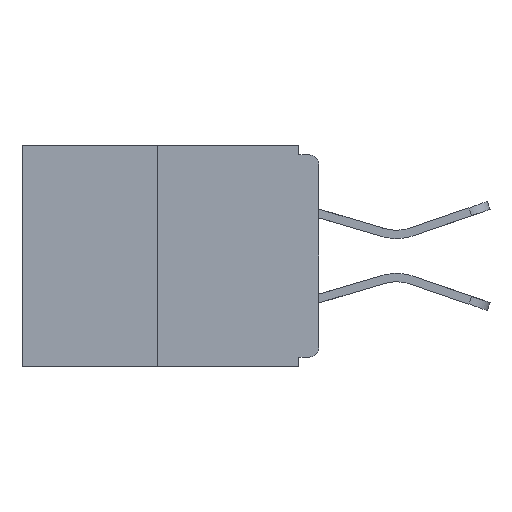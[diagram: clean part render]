
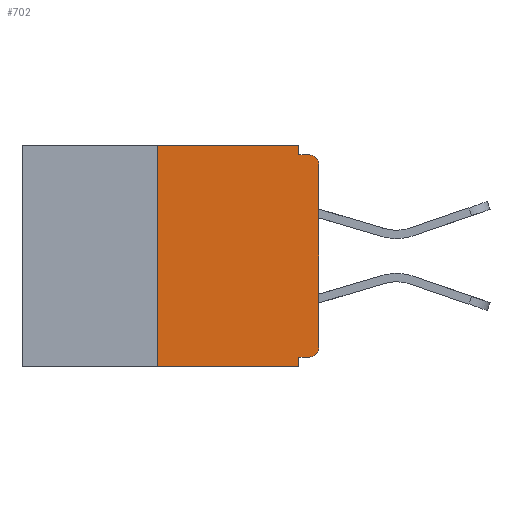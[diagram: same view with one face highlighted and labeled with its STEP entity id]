
A CAD part, left-side view. The second image highlights one B-rep face of the part: STEP entity #702.
In plain terms, the highlighted planar face has unit normal (-1, 0, 0).
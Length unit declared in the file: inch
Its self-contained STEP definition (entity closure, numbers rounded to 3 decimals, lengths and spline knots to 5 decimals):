
#124 = ORIENTED_EDGE ( 'NONE', *, *, #10964, .F. ) ;
#320 = VERTEX_POINT ( 'NONE', #9749 ) ;
#351 = PLANE ( 'NONE',  #2901 ) ;
#610 = ORIENTED_EDGE ( 'NONE', *, *, #4471, .F. ) ;
#689 = CARTESIAN_POINT ( 'NONE',  ( 0., 0., 0. ) ) ;
#702 = ADVANCED_FACE ( 'NONE', ( #7585 ), #351, .F. ) ;
#805 = VERTEX_POINT ( 'NONE', #10018 ) ;
#1058 = CARTESIAN_POINT ( 'NONE',  ( 0., 0.015, -0.313 ) ) ;
#1541 = VECTOR ( 'NONE', #9274, 39.37008 ) ;
#1599 = LINE ( 'NONE', #11029, #1541 ) ;
#1915 = LINE ( 'NONE', #8311, #6901 ) ;
#1949 = DIRECTION ( 'NONE',  ( 0., -1., 0. ) ) ;
#2059 = VERTEX_POINT ( 'NONE', #11018 ) ;
#2078 = EDGE_CURVE ( 'NONE', #9337, #805, #11120, .T. ) ;
#2152 = DIRECTION ( 'NONE',  ( 0., -1., 0. ) ) ;
#2305 = VERTEX_POINT ( 'NONE', #6916 ) ;
#2312 = VECTOR ( 'NONE', #1949, 39.37008 ) ;
#2346 = CARTESIAN_POINT ( 'NONE',  ( 0., 0., -0.313 ) ) ;
#2625 = ORIENTED_EDGE ( 'NONE', *, *, #2078, .F. ) ;
#2716 = CARTESIAN_POINT ( 'NONE',  ( 0., 0., -0.328 ) ) ;
#2770 = VECTOR ( 'NONE', #9313, 39.37008 ) ;
#2778 = ORIENTED_EDGE ( 'NONE', *, *, #6519, .T. ) ;
#2830 = CARTESIAN_POINT ( 'NONE',  ( 0., 0.46, 0. ) ) ;
#2896 = VECTOR ( 'NONE', #4138, 39.37008 ) ;
#2901 = AXIS2_PLACEMENT_3D ( 'NONE', #7775, #10579, #3884 ) ;
#3546 = DIRECTION ( 'NONE',  ( 0., 0., -1. ) ) ;
#3884 = DIRECTION ( 'NONE',  ( 0., 0., -1. ) ) ;
#3904 = AXIS2_PLACEMENT_3D ( 'NONE', #1058, #10192, #11138 ) ;
#4128 = EDGE_CURVE ( 'NONE', #8299, #6694, #10891, .T. ) ;
#4138 = DIRECTION ( 'NONE',  ( 0., 0., 1. ) ) ;
#4146 = VERTEX_POINT ( 'NONE', #9282 ) ;
#4350 = ORIENTED_EDGE ( 'NONE', *, *, #9958, .F. ) ;
#4471 = EDGE_CURVE ( 'NONE', #8299, #320, #11007, .T. ) ;
#4793 = ORIENTED_EDGE ( 'NONE', *, *, #5158, .F. ) ;
#5037 = CARTESIAN_POINT ( 'NONE',  ( 0., 0.031, -0.015 ) ) ;
#5158 = EDGE_CURVE ( 'NONE', #2059, #9337, #1599, .T. ) ;
#5454 = LINE ( 'NONE', #8080, #9837 ) ;
#5830 = EDGE_CURVE ( 'NONE', #6694, #4146, #8707, .T. ) ;
#6205 = CARTESIAN_POINT ( 'NONE',  ( 0., 0.25, 0. ) ) ;
#6346 = EDGE_CURVE ( 'NONE', #9575, #2305, #10578, .T. ) ;
#6460 = AXIS2_PLACEMENT_3D ( 'NONE', #7509, #6597, #9516 ) ;
#6473 = LINE ( 'NONE', #11143, #6824 ) ;
#6519 = EDGE_CURVE ( 'NONE', #4146, #2305, #7239, .T. ) ;
#6597 = DIRECTION ( 'NONE',  ( -1., 0., 0. ) ) ;
#6627 = EDGE_CURVE ( 'NONE', #2059, #10246, #6473, .T. ) ;
#6694 = VERTEX_POINT ( 'NONE', #2346 ) ;
#6824 = VECTOR ( 'NONE', #2152, 39.37008 ) ;
#6901 = VECTOR ( 'NONE', #8415, 39.37008 ) ;
#6916 = CARTESIAN_POINT ( 'NONE',  ( 0., 0.015, -0.015 ) ) ;
#7239 = CIRCLE ( 'NONE', #6460, 0.015 ) ;
#7421 = VECTOR ( 'NONE', #10756, 39.37008 ) ;
#7509 = CARTESIAN_POINT ( 'NONE',  ( 0., 0.015, -0.03 ) ) ;
#7546 = ORIENTED_EDGE ( 'NONE', *, *, #4128, .T. ) ;
#7585 = FACE_OUTER_BOUND ( 'NONE', #11859, .T. ) ;
#7775 = CARTESIAN_POINT ( 'NONE',  ( 0., 0.46, 0. ) ) ;
#7832 = CARTESIAN_POINT ( 'NONE',  ( 0., 0., -0.015 ) ) ;
#8080 = CARTESIAN_POINT ( 'NONE',  ( 0., 0.031, 0. ) ) ;
#8225 = ORIENTED_EDGE ( 'NONE', *, *, #6627, .T. ) ;
#8299 = VERTEX_POINT ( 'NONE', #10341 ) ;
#8311 = CARTESIAN_POINT ( 'NONE',  ( 0., 0.031, -0.343 ) ) ;
#8415 = DIRECTION ( 'NONE',  ( 0., 0., -1. ) ) ;
#8707 = LINE ( 'NONE', #689, #2896 ) ;
#9274 = DIRECTION ( 'NONE',  ( 0., 0., 1. ) ) ;
#9282 = CARTESIAN_POINT ( 'NONE',  ( 0., 0., -0.03 ) ) ;
#9313 = DIRECTION ( 'NONE',  ( 0., 1., 0. ) ) ;
#9337 = VERTEX_POINT ( 'NONE', #6205 ) ;
#9516 = DIRECTION ( 'NONE',  ( 0., 0., -1. ) ) ;
#9575 = VERTEX_POINT ( 'NONE', #5037 ) ;
#9749 = CARTESIAN_POINT ( 'NONE',  ( 0., 0.031, -0.328 ) ) ;
#9837 = VECTOR ( 'NONE', #3546, 39.37008 ) ;
#9958 = EDGE_CURVE ( 'NONE', #320, #10246, #1915, .T. ) ;
#10018 = CARTESIAN_POINT ( 'NONE',  ( 0., 0.031, 0. ) ) ;
#10192 = DIRECTION ( 'NONE',  ( -1., 0., 0. ) ) ;
#10246 = VERTEX_POINT ( 'NONE', #10744 ) ;
#10341 = CARTESIAN_POINT ( 'NONE',  ( 0., 0.015, -0.328 ) ) ;
#10490 = ORIENTED_EDGE ( 'NONE', *, *, #6346, .F. ) ;
#10578 = LINE ( 'NONE', #7832, #7421 ) ;
#10579 = DIRECTION ( 'NONE',  ( 1., 0., 0. ) ) ;
#10604 = ORIENTED_EDGE ( 'NONE', *, *, #5830, .T. ) ;
#10744 = CARTESIAN_POINT ( 'NONE',  ( 0., 0.031, -0.343 ) ) ;
#10756 = DIRECTION ( 'NONE',  ( 0., -1., 0. ) ) ;
#10891 = CIRCLE ( 'NONE', #3904, 0.015 ) ;
#10964 = EDGE_CURVE ( 'NONE', #805, #9575, #5454, .T. ) ;
#11007 = LINE ( 'NONE', #2716, #2770 ) ;
#11018 = CARTESIAN_POINT ( 'NONE',  ( 0., 0.25, -0.343 ) ) ;
#11029 = CARTESIAN_POINT ( 'NONE',  ( 0., 0.25, 0. ) ) ;
#11120 = LINE ( 'NONE', #2830, #2312 ) ;
#11138 = DIRECTION ( 'NONE',  ( 0., 0., -1. ) ) ;
#11143 = CARTESIAN_POINT ( 'NONE',  ( 0., 0.46, -0.343 ) ) ;
#11859 = EDGE_LOOP ( 'NONE', ( #2625, #4793, #8225, #4350, #610, #7546, #10604, #2778, #10490, #124 ) ) ;
